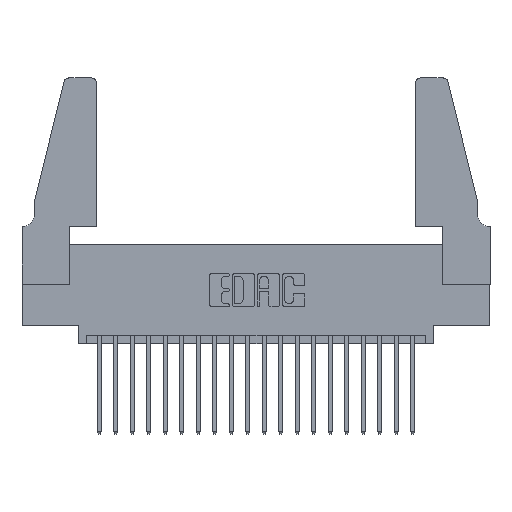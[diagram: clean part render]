
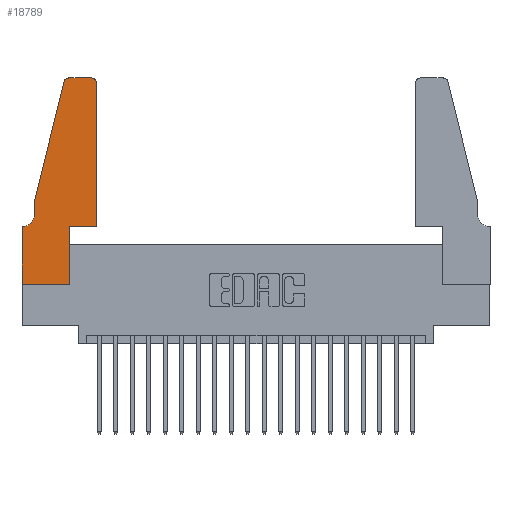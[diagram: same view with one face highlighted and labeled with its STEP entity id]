
A CAD part, top view. The second image highlights one B-rep face of the part: STEP entity #18789.
In plain terms, the highlighted planar face has unit normal (0, 0, 1).
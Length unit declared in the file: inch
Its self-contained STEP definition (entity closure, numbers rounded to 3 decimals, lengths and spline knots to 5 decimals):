
#25 = CARTESIAN_POINT ( 'NONE',  ( 0., 0.35, 0.37 ) ) ;
#93 = ORIENTED_EDGE ( 'NONE', *, *, #19586, .T. ) ;
#682 = DIRECTION ( 'NONE',  ( 0., 0., 1. ) ) ;
#919 = FACE_OUTER_BOUND ( 'NONE', #5402, .T. ) ;
#1090 = ORIENTED_EDGE ( 'NONE', *, *, #1647, .T. ) ;
#1465 = ORIENTED_EDGE ( 'NONE', *, *, #17004, .T. ) ;
#1529 = DIRECTION ( 'NONE',  ( 0., -1., 0. ) ) ;
#1549 = DIRECTION ( 'NONE',  ( 0., 1., 0. ) ) ;
#1557 = LINE ( 'NONE', #6458, #5434 ) ;
#1647 = EDGE_CURVE ( 'NONE', #16497, #14474, #11501, .T. ) ;
#1759 = DIRECTION ( 'NONE',  ( 1., 0., 0. ) ) ;
#1957 = EDGE_CURVE ( 'NONE', #2903, #12718, #5818, .T. ) ;
#2087 = CARTESIAN_POINT ( 'NONE',  ( 0.0755, 0.5, 0.37 ) ) ;
#2710 = VERTEX_POINT ( 'NONE', #16353 ) ;
#2903 = VERTEX_POINT ( 'NONE', #19042 ) ;
#3128 = CIRCLE ( 'NONE', #15265, 0.03 ) ;
#3302 = AXIS2_PLACEMENT_3D ( 'NONE', #18289, #4213, #3784 ) ;
#3423 = VECTOR ( 'NONE', #4309, 39.37008 ) ;
#3587 = LINE ( 'NONE', #8296, #18028 ) ;
#3784 = DIRECTION ( 'NONE',  ( -1., 0., 0. ) ) ;
#4213 = DIRECTION ( 'NONE',  ( 0., 0., -1. ) ) ;
#4309 = DIRECTION ( 'NONE',  ( -1., 0., 0. ) ) ;
#4334 = LINE ( 'NONE', #19213, #16748 ) ;
#4351 = DIRECTION ( 'NONE',  ( 0., 0., 1. ) ) ;
#4494 = CARTESIAN_POINT ( 'NONE',  ( 0.4205, 1.25, 0.37 ) ) ;
#4547 = ORIENTED_EDGE ( 'NONE', *, *, #5064, .T. ) ;
#4624 = CARTESIAN_POINT ( 'NONE',  ( 0., 0.35, 0.37 ) ) ;
#5064 = EDGE_CURVE ( 'NONE', #2710, #15686, #3128, .T. ) ;
#5258 = EDGE_CURVE ( 'NONE', #15686, #5675, #16340, .T. ) ;
#5390 = EDGE_CURVE ( 'NONE', #13278, #8081, #10116, .T. ) ;
#5402 = EDGE_LOOP ( 'NONE', ( #20546, #18991, #10537, #93, #1090, #11365, #8569, #12706, #16409, #11326, #1465, #4547 ) ) ;
#5434 = VECTOR ( 'NONE', #1549, 39.37008 ) ;
#5675 = VERTEX_POINT ( 'NONE', #20257 ) ;
#5788 = LINE ( 'NONE', #2087, #7336 ) ;
#5818 = LINE ( 'NONE', #12751, #18175 ) ;
#6149 = DIRECTION ( 'NONE',  ( -1., 0., 0. ) ) ;
#6458 = CARTESIAN_POINT ( 'NONE',  ( 0.4505, 0.35, 0.37 ) ) ;
#7058 = EDGE_CURVE ( 'NONE', #7548, #10382, #13054, .T. ) ;
#7336 = VECTOR ( 'NONE', #13563, 39.37008 ) ;
#7548 = VERTEX_POINT ( 'NONE', #13721 ) ;
#7621 = CARTESIAN_POINT ( 'NONE',  ( 0.4505, 0.35, 0.37 ) ) ;
#8081 = VERTEX_POINT ( 'NONE', #14946 ) ;
#8296 = CARTESIAN_POINT ( 'NONE',  ( 0., 0., 0.37 ) ) ;
#8302 = VECTOR ( 'NONE', #6149, 39.37008 ) ;
#8349 = PLANE ( 'NONE',  #19118 ) ;
#8351 = LINE ( 'NONE', #9245, #3423 ) ;
#8569 = ORIENTED_EDGE ( 'NONE', *, *, #5390, .T. ) ;
#8759 = VECTOR ( 'NONE', #18897, 39.37008 ) ;
#9245 = CARTESIAN_POINT ( 'NONE',  ( 0.0755, 0.35, 0.37 ) ) ;
#9598 = VECTOR ( 'NONE', #1529, 39.37008 ) ;
#9941 = CARTESIAN_POINT ( 'NONE',  ( 0.4505, 0.35, 0.37 ) ) ;
#9967 = DIRECTION ( 'NONE',  ( 1., 0., 0. ) ) ;
#10116 = LINE ( 'NONE', #13021, #9598 ) ;
#10382 = VERTEX_POINT ( 'NONE', #9941 ) ;
#10537 = ORIENTED_EDGE ( 'NONE', *, *, #1957, .T. ) ;
#10579 = CARTESIAN_POINT ( 'NONE',  ( 0.4205, 1.22, 0.37 ) ) ;
#11326 = ORIENTED_EDGE ( 'NONE', *, *, #7058, .T. ) ;
#11360 = CIRCLE ( 'NONE', #12242, 0.03 ) ;
#11365 = ORIENTED_EDGE ( 'NONE', *, *, #20367, .T. ) ;
#11501 = CIRCLE ( 'NONE', #3302, 0.07 ) ;
#11515 = CARTESIAN_POINT ( 'NONE',  ( 0.2865, 0., 0.37 ) ) ;
#11606 = EDGE_CURVE ( 'NONE', #8081, #16482, #3587, .T. ) ;
#11632 = DIRECTION ( 'NONE',  ( 0., 0., 1. ) ) ;
#12021 = DIRECTION ( 'NONE',  ( -0.239, -0.971, 0. ) ) ;
#12211 = DIRECTION ( 'NONE',  ( 1., 0., 0. ) ) ;
#12242 = AXIS2_PLACEMENT_3D ( 'NONE', #14141, #4351, #15724 ) ;
#12706 = ORIENTED_EDGE ( 'NONE', *, *, #11606, .T. ) ;
#12718 = VERTEX_POINT ( 'NONE', #13161 ) ;
#12751 = CARTESIAN_POINT ( 'NONE',  ( 0.0755, 0.5, 0.37 ) ) ;
#13021 = CARTESIAN_POINT ( 'NONE',  ( 0., 0., 0.37 ) ) ;
#13054 = LINE ( 'NONE', #7621, #8759 ) ;
#13161 = CARTESIAN_POINT ( 'NONE',  ( 0.0755, 0.5, 0.37 ) ) ;
#13278 = VERTEX_POINT ( 'NONE', #4624 ) ;
#13563 = DIRECTION ( 'NONE',  ( 0., -1., 0. ) ) ;
#13721 = CARTESIAN_POINT ( 'NONE',  ( 0.2865, 0.35, 0.37 ) ) ;
#14141 = CARTESIAN_POINT ( 'NONE',  ( 0.284, 1.22, 0.37 ) ) ;
#14474 = VERTEX_POINT ( 'NONE', #15664 ) ;
#14550 = DIRECTION ( 'NONE',  ( 0., 1., 0. ) ) ;
#14946 = CARTESIAN_POINT ( 'NONE',  ( 0., 0., 0.37 ) ) ;
#15265 = AXIS2_PLACEMENT_3D ( 'NONE', #10579, #682, #12211 ) ;
#15664 = CARTESIAN_POINT ( 'NONE',  ( 0.0055, 0.35, 0.37 ) ) ;
#15686 = VERTEX_POINT ( 'NONE', #4494 ) ;
#15724 = DIRECTION ( 'NONE',  ( 1., 0., 0. ) ) ;
#15860 = CARTESIAN_POINT ( 'NONE',  ( 0.2605, 1.25, 0.37 ) ) ;
#16340 = LINE ( 'NONE', #15860, #8302 ) ;
#16353 = CARTESIAN_POINT ( 'NONE',  ( 0.4505, 1.22, 0.37 ) ) ;
#16409 = ORIENTED_EDGE ( 'NONE', *, *, #17587, .T. ) ;
#16482 = VERTEX_POINT ( 'NONE', #11515 ) ;
#16497 = VERTEX_POINT ( 'NONE', #17885 ) ;
#16748 = VECTOR ( 'NONE', #14550, 39.37008 ) ;
#17004 = EDGE_CURVE ( 'NONE', #10382, #2710, #1557, .T. ) ;
#17418 = EDGE_CURVE ( 'NONE', #5675, #2903, #11360, .T. ) ;
#17587 = EDGE_CURVE ( 'NONE', #16482, #7548, #4334, .T. ) ;
#17885 = CARTESIAN_POINT ( 'NONE',  ( 0.0755, 0.42, 0.37 ) ) ;
#18028 = VECTOR ( 'NONE', #9967, 39.37008 ) ;
#18175 = VECTOR ( 'NONE', #12021, 39.37008 ) ;
#18289 = CARTESIAN_POINT ( 'NONE',  ( 0.0055, 0.42, 0.37 ) ) ;
#18789 = ADVANCED_FACE ( 'NONE', ( #919 ), #8349, .T. ) ;
#18897 = DIRECTION ( 'NONE',  ( 1., 0., 0. ) ) ;
#18991 = ORIENTED_EDGE ( 'NONE', *, *, #17418, .T. ) ;
#19042 = CARTESIAN_POINT ( 'NONE',  ( 0.25487, 1.22718, 0.37 ) ) ;
#19118 = AXIS2_PLACEMENT_3D ( 'NONE', #25, #11632, #1759 ) ;
#19213 = CARTESIAN_POINT ( 'NONE',  ( 0.2865, 0.35, 0.37 ) ) ;
#19586 = EDGE_CURVE ( 'NONE', #12718, #16497, #5788, .T. ) ;
#20257 = CARTESIAN_POINT ( 'NONE',  ( 0.284, 1.25, 0.37 ) ) ;
#20367 = EDGE_CURVE ( 'NONE', #14474, #13278, #8351, .T. ) ;
#20546 = ORIENTED_EDGE ( 'NONE', *, *, #5258, .T. ) ;
